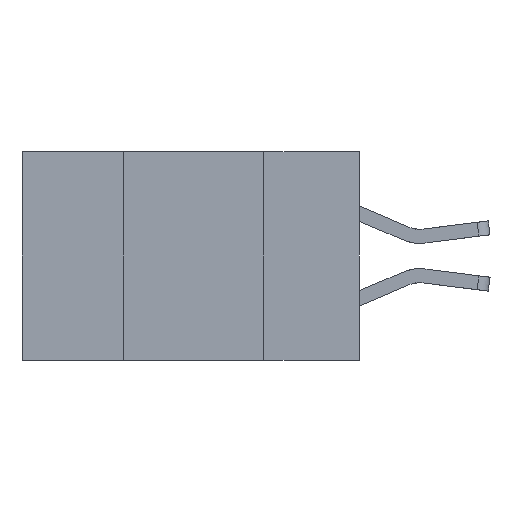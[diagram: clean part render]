
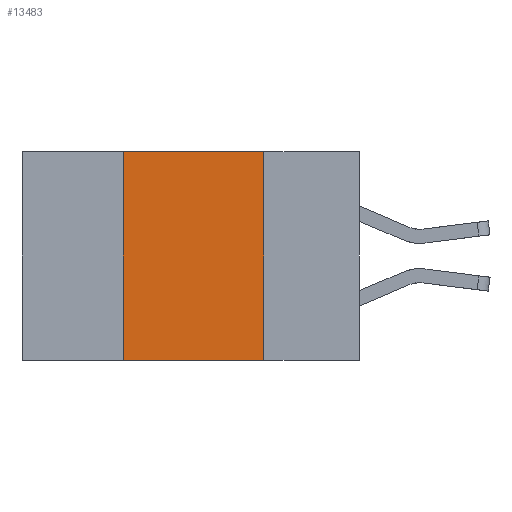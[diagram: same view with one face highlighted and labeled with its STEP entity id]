
A CAD part, left-side view. The second image highlights one B-rep face of the part: STEP entity #13483.
In plain terms, the highlighted planar face has unit normal (-1, 0, 0).
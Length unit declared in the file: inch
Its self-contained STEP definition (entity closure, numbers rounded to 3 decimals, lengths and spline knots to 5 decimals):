
#412 = VERTEX_POINT ( 'NONE', #12074 ) ;
#700 = EDGE_CURVE ( 'NONE', #412, #11526, #11404, .T. ) ;
#1163 = CARTESIAN_POINT ( 'NONE',  ( 0., 0.6, -0.37 ) ) ;
#1616 = EDGE_CURVE ( 'NONE', #13943, #11526, #9010, .T. ) ;
#2022 = CARTESIAN_POINT ( 'NONE',  ( 0., 0.42, -0.37 ) ) ;
#2131 = CARTESIAN_POINT ( 'NONE',  ( 0., 0.17, -0.37 ) ) ;
#2452 = DIRECTION ( 'NONE',  ( 0., 0., -1. ) ) ;
#2686 = DIRECTION ( 'NONE',  ( 0., 0., 1. ) ) ;
#3411 = DIRECTION ( 'NONE',  ( 0., -1., 0. ) ) ;
#3877 = VECTOR ( 'NONE', #11648, 39.37008 ) ;
#4416 = VECTOR ( 'NONE', #12878, 39.37008 ) ;
#4667 = AXIS2_PLACEMENT_3D ( 'NONE', #4835, #12999, #2452 ) ;
#4835 = CARTESIAN_POINT ( 'NONE',  ( 0., 0.6, 0. ) ) ;
#4849 = ORIENTED_EDGE ( 'NONE', *, *, #1616, .T. ) ;
#5233 = EDGE_CURVE ( 'NONE', #8711, #412, #11290, .T. ) ;
#5635 = ORIENTED_EDGE ( 'NONE', *, *, #14202, .F. ) ;
#6507 = VECTOR ( 'NONE', #2686, 39.37008 ) ;
#6918 = CARTESIAN_POINT ( 'NONE',  ( 0., 0.17, 0. ) ) ;
#7087 = FACE_OUTER_BOUND ( 'NONE', #8743, .T. ) ;
#7187 = PLANE ( 'NONE',  #4667 ) ;
#8018 = CARTESIAN_POINT ( 'NONE',  ( 0., 0.42, 0. ) ) ;
#8195 = LINE ( 'NONE', #10750, #6507 ) ;
#8711 = VERTEX_POINT ( 'NONE', #8018 ) ;
#8743 = EDGE_LOOP ( 'NONE', ( #12101, #10992, #5635, #4849 ) ) ;
#9010 = LINE ( 'NONE', #1163, #4416 ) ;
#10414 = CARTESIAN_POINT ( 'NONE',  ( 0., 0.6, 0. ) ) ;
#10750 = CARTESIAN_POINT ( 'NONE',  ( 0., 0.42, 0. ) ) ;
#10992 = ORIENTED_EDGE ( 'NONE', *, *, #5233, .F. ) ;
#11290 = LINE ( 'NONE', #10414, #11647 ) ;
#11404 = LINE ( 'NONE', #6918, #3877 ) ;
#11526 = VERTEX_POINT ( 'NONE', #2131 ) ;
#11647 = VECTOR ( 'NONE', #3411, 39.37008 ) ;
#11648 = DIRECTION ( 'NONE',  ( 0., 0., -1. ) ) ;
#12074 = CARTESIAN_POINT ( 'NONE',  ( 0., 0.17, 0. ) ) ;
#12101 = ORIENTED_EDGE ( 'NONE', *, *, #700, .F. ) ;
#12878 = DIRECTION ( 'NONE',  ( 0., -1., 0. ) ) ;
#12999 = DIRECTION ( 'NONE',  ( 1., 0., 0. ) ) ;
#13483 = ADVANCED_FACE ( 'NONE', ( #7087 ), #7187, .F. ) ;
#13943 = VERTEX_POINT ( 'NONE', #2022 ) ;
#14202 = EDGE_CURVE ( 'NONE', #13943, #8711, #8195, .T. ) ;
